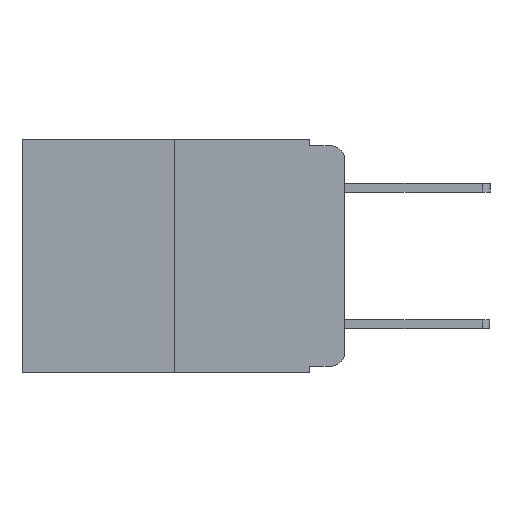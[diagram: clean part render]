
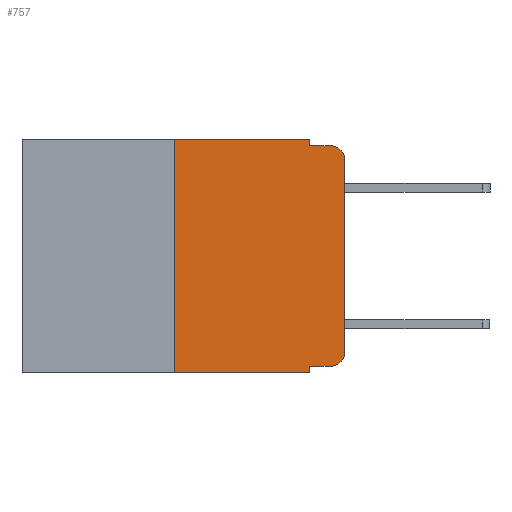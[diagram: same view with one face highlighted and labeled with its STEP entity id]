
A CAD part, left-side view. The second image highlights one B-rep face of the part: STEP entity #757.
In plain terms, the highlighted planar face has unit normal (-1, 0, 0).
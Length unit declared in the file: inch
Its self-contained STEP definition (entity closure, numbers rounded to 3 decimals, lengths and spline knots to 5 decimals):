
#34 = VERTEX_POINT ( 'NONE', #17705 ) ;
#80 = LINE ( 'NONE', #13789, #15010 ) ;
#291 = VERTEX_POINT ( 'NONE', #10884 ) ;
#617 = CIRCLE ( 'NONE', #4133, 0.02 ) ;
#757 = ADVANCED_FACE ( 'NONE', ( #15026 ), #11151, .F. ) ;
#892 = VERTEX_POINT ( 'NONE', #14656 ) ;
#1216 = EDGE_LOOP ( 'NONE', ( #3423, #2980, #2473, #3541, #3038, #14312, #17909, #4606, #5634, #2247 ) ) ;
#1427 = CARTESIAN_POINT ( 'NONE',  ( 0., 0.051, 0. ) ) ;
#1623 = VERTEX_POINT ( 'NONE', #12191 ) ;
#1942 = CIRCLE ( 'NONE', #14378, 0.02 ) ;
#2247 = ORIENTED_EDGE ( 'NONE', *, *, #4053, .T. ) ;
#2286 = VECTOR ( 'NONE', #13170, 39.37008 ) ;
#2473 = ORIENTED_EDGE ( 'NONE', *, *, #3982, .F. ) ;
#2815 = LINE ( 'NONE', #17961, #2286 ) ;
#2980 = ORIENTED_EDGE ( 'NONE', *, *, #3981, .T. ) ;
#3038 = ORIENTED_EDGE ( 'NONE', *, *, #3145, .F. ) ;
#3145 = EDGE_CURVE ( 'NONE', #6138, #12170, #2815, .T. ) ;
#3423 = ORIENTED_EDGE ( 'NONE', *, *, #3977, .T. ) ;
#3541 = ORIENTED_EDGE ( 'NONE', *, *, #4016, .F. ) ;
#3601 = EDGE_CURVE ( 'NONE', #892, #14857, #5366, .T. ) ;
#3977 = EDGE_CURVE ( 'NONE', #6117, #34, #12519, .T. ) ;
#3981 = EDGE_CURVE ( 'NONE', #34, #1623, #617, .T. ) ;
#3982 = EDGE_CURVE ( 'NONE', #13634, #1623, #80, .T. ) ;
#4008 = DIRECTION ( 'NONE',  ( 0., -1., 0. ) ) ;
#4016 = EDGE_CURVE ( 'NONE', #12170, #13634, #10977, .T. ) ;
#4021 = EDGE_CURVE ( 'NONE', #892, #6138, #14264, .T. ) ;
#4046 = EDGE_CURVE ( 'NONE', #9338, #14857, #17111, .T. ) ;
#4051 = EDGE_CURVE ( 'NONE', #9338, #291, #13493, .T. ) ;
#4053 = EDGE_CURVE ( 'NONE', #291, #6117, #1942, .T. ) ;
#4133 = AXIS2_PLACEMENT_3D ( 'NONE', #16260, #8642, #17479 ) ;
#4606 = ORIENTED_EDGE ( 'NONE', *, *, #4046, .F. ) ;
#5366 = LINE ( 'NONE', #6708, #12360 ) ;
#5634 = ORIENTED_EDGE ( 'NONE', *, *, #4051, .T. ) ;
#6117 = VERTEX_POINT ( 'NONE', #17367 ) ;
#6138 = VERTEX_POINT ( 'NONE', #10015 ) ;
#6193 = CARTESIAN_POINT ( 'NONE',  ( 0., 0.473, 0. ) ) ;
#6708 = CARTESIAN_POINT ( 'NONE',  ( 0., 0.473, -0.343 ) ) ;
#7239 = VECTOR ( 'NONE', #8764, 39.37008 ) ;
#7441 = DIRECTION ( 'NONE',  ( 0., 0., -1. ) ) ;
#7510 = CARTESIAN_POINT ( 'NONE',  ( 0., 0.02, -0.313 ) ) ;
#8070 = AXIS2_PLACEMENT_3D ( 'NONE', #6193, #15222, #7441 ) ;
#8134 = DIRECTION ( 'NONE',  ( 0., -1., 0. ) ) ;
#8587 = VECTOR ( 'NONE', #9964, 39.37008 ) ;
#8642 = DIRECTION ( 'NONE',  ( -1., 0., 0. ) ) ;
#8657 = CARTESIAN_POINT ( 'NONE',  ( 0., 0.051, -0.333 ) ) ;
#8764 = DIRECTION ( 'NONE',  ( 0., 0., -1. ) ) ;
#8933 = DIRECTION ( 'NONE',  ( 0., 0., -1. ) ) ;
#9338 = VERTEX_POINT ( 'NONE', #8657 ) ;
#9964 = DIRECTION ( 'NONE',  ( 0., 0., 1. ) ) ;
#10015 = CARTESIAN_POINT ( 'NONE',  ( 0., 0.25, 0. ) ) ;
#10548 = VECTOR ( 'NONE', #15225, 39.37008 ) ;
#10884 = CARTESIAN_POINT ( 'NONE',  ( 0., 0.02, -0.333 ) ) ;
#10977 = LINE ( 'NONE', #13907, #7239 ) ;
#11151 = PLANE ( 'NONE',  #8070 ) ;
#11311 = CARTESIAN_POINT ( 'NONE',  ( 0., 0.051, -0.01 ) ) ;
#11582 = DIRECTION ( 'NONE',  ( 0., -1., 0. ) ) ;
#12170 = VERTEX_POINT ( 'NONE', #1427 ) ;
#12191 = CARTESIAN_POINT ( 'NONE',  ( 0., 0.02, -0.01 ) ) ;
#12291 = CARTESIAN_POINT ( 'NONE',  ( 0., 0.051, -0.343 ) ) ;
#12360 = VECTOR ( 'NONE', #8134, 39.37008 ) ;
#12519 = LINE ( 'NONE', #13745, #8587 ) ;
#12671 = DIRECTION ( 'NONE',  ( 0., 0., 1. ) ) ;
#13094 = VECTOR ( 'NONE', #11582, 39.37008 ) ;
#13170 = DIRECTION ( 'NONE',  ( 0., -1., 0. ) ) ;
#13493 = LINE ( 'NONE', #16469, #13094 ) ;
#13634 = VERTEX_POINT ( 'NONE', #11311 ) ;
#13745 = CARTESIAN_POINT ( 'NONE',  ( 0., 0., 0. ) ) ;
#13789 = CARTESIAN_POINT ( 'NONE',  ( 0., 0.051, -0.01 ) ) ;
#13907 = CARTESIAN_POINT ( 'NONE',  ( 0., 0.051, 0. ) ) ;
#14264 = LINE ( 'NONE', #17579, #14649 ) ;
#14312 = ORIENTED_EDGE ( 'NONE', *, *, #4021, .F. ) ;
#14378 = AXIS2_PLACEMENT_3D ( 'NONE', #7510, #16522, #8933 ) ;
#14649 = VECTOR ( 'NONE', #12671, 39.37008 ) ;
#14656 = CARTESIAN_POINT ( 'NONE',  ( 0., 0.25, -0.343 ) ) ;
#14857 = VERTEX_POINT ( 'NONE', #12291 ) ;
#15010 = VECTOR ( 'NONE', #4008, 39.37008 ) ;
#15026 = FACE_OUTER_BOUND ( 'NONE', #1216, .T. ) ;
#15222 = DIRECTION ( 'NONE',  ( 1., 0., 0. ) ) ;
#15225 = DIRECTION ( 'NONE',  ( 0., 0., -1. ) ) ;
#16260 = CARTESIAN_POINT ( 'NONE',  ( 0., 0.02, -0.03 ) ) ;
#16469 = CARTESIAN_POINT ( 'NONE',  ( 0., 0.051, -0.333 ) ) ;
#16522 = DIRECTION ( 'NONE',  ( -1., 0., 0. ) ) ;
#17111 = LINE ( 'NONE', #17685, #10548 ) ;
#17367 = CARTESIAN_POINT ( 'NONE',  ( 0., 0., -0.313 ) ) ;
#17479 = DIRECTION ( 'NONE',  ( 0., 0., -1. ) ) ;
#17579 = CARTESIAN_POINT ( 'NONE',  ( 0., 0.25, 0. ) ) ;
#17685 = CARTESIAN_POINT ( 'NONE',  ( 0., 0.051, 0. ) ) ;
#17705 = CARTESIAN_POINT ( 'NONE',  ( 0., 0., -0.03 ) ) ;
#17909 = ORIENTED_EDGE ( 'NONE', *, *, #3601, .T. ) ;
#17961 = CARTESIAN_POINT ( 'NONE',  ( 0., 0.473, 0. ) ) ;
